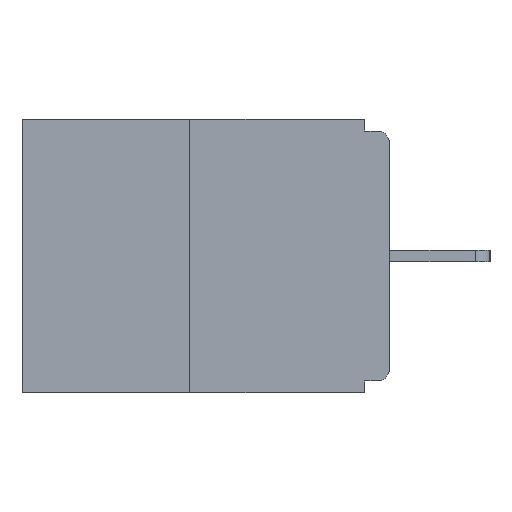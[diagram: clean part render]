
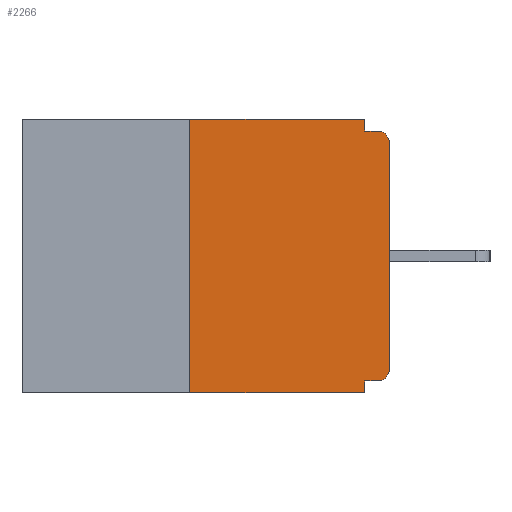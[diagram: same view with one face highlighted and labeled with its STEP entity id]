
A CAD part, left-side view. The second image highlights one B-rep face of the part: STEP entity #2266.
In plain terms, the highlighted planar face has unit normal (-1, 0, 0).
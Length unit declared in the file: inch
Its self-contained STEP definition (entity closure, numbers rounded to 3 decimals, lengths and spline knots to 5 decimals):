
#65 = EDGE_CURVE ( 'NONE', #19768, #17656, #17160, .T. ) ;
#498 = VERTEX_POINT ( 'NONE', #9964 ) ;
#1561 = DIRECTION ( 'NONE',  ( 0., 0., 1. ) ) ;
#2215 = ORIENTED_EDGE ( 'NONE', *, *, #4279, .T. ) ;
#2250 = VERTEX_POINT ( 'NONE', #8593 ) ;
#2266 = ADVANCED_FACE ( 'NONE', ( #8035 ), #17076, .F. ) ;
#3750 = EDGE_CURVE ( 'NONE', #2250, #498, #4359, .T. ) ;
#3853 = CARTESIAN_POINT ( 'NONE',  ( 0., 0.031, -0.328 ) ) ;
#3857 = DIRECTION ( 'NONE',  ( 1., 0., 0. ) ) ;
#4024 = AXIS2_PLACEMENT_3D ( 'NONE', #25520, #3857, #18879 ) ;
#4279 = EDGE_CURVE ( 'NONE', #18692, #2250, #9939, .T. ) ;
#4333 = EDGE_CURVE ( 'NONE', #14753, #22652, #13952, .T. ) ;
#4359 = CIRCLE ( 'NONE', #23442, 0.015 ) ;
#4551 = CARTESIAN_POINT ( 'NONE',  ( 0., 0., -0.015 ) ) ;
#4569 = EDGE_CURVE ( 'NONE', #14753, #17118, #5358, .T. ) ;
#4645 = EDGE_CURVE ( 'NONE', #17656, #498, #15135, .T. ) ;
#4673 = DIRECTION ( 'NONE',  ( -1., 0., 0. ) ) ;
#5358 = LINE ( 'NONE', #18330, #16076 ) ;
#5382 = VECTOR ( 'NONE', #1561, 39.37008 ) ;
#5445 = CARTESIAN_POINT ( 'NONE',  ( 0., 0.015, -0.313 ) ) ;
#6482 = CARTESIAN_POINT ( 'NONE',  ( 0., 0.46, 0. ) ) ;
#6751 = CARTESIAN_POINT ( 'NONE',  ( 0., 0.031, -0.343 ) ) ;
#7049 = CARTESIAN_POINT ( 'NONE',  ( 0., 0.25, -0.343 ) ) ;
#7251 = CARTESIAN_POINT ( 'NONE',  ( 0., 0.015, -0.328 ) ) ;
#7298 = DIRECTION ( 'NONE',  ( 0., 0., 1. ) ) ;
#7662 = ORIENTED_EDGE ( 'NONE', *, *, #65, .F. ) ;
#8035 = FACE_OUTER_BOUND ( 'NONE', #9045, .T. ) ;
#8593 = CARTESIAN_POINT ( 'NONE',  ( 0., 0., -0.03 ) ) ;
#8756 = ORIENTED_EDGE ( 'NONE', *, *, #3750, .T. ) ;
#9045 = EDGE_LOOP ( 'NONE', ( #25460, #13116, #10959, #24243, #26529, #23809, #2215, #8756, #13573, #7662 ) ) ;
#9939 = LINE ( 'NONE', #20631, #5382 ) ;
#9964 = CARTESIAN_POINT ( 'NONE',  ( 0., 0.015, -0.015 ) ) ;
#10185 = CARTESIAN_POINT ( 'NONE',  ( 0., 0.031, 0. ) ) ;
#10533 = LINE ( 'NONE', #6482, #20190 ) ;
#10557 = CIRCLE ( 'NONE', #19886, 0.015 ) ;
#10936 = DIRECTION ( 'NONE',  ( 0., 0., -1. ) ) ;
#10959 = ORIENTED_EDGE ( 'NONE', *, *, #4333, .T. ) ;
#12269 = DIRECTION ( 'NONE',  ( 0., -1., 0. ) ) ;
#12533 = CARTESIAN_POINT ( 'NONE',  ( 0., 0.25, 0. ) ) ;
#12976 = DIRECTION ( 'NONE',  ( 0., 1., 0. ) ) ;
#13116 = ORIENTED_EDGE ( 'NONE', *, *, #4569, .F. ) ;
#13355 = VECTOR ( 'NONE', #21061, 39.37008 ) ;
#13573 = ORIENTED_EDGE ( 'NONE', *, *, #4645, .F. ) ;
#13926 = DIRECTION ( 'NONE',  ( 0., 0., -1. ) ) ;
#13952 = LINE ( 'NONE', #14377, #16057 ) ;
#14137 = EDGE_CURVE ( 'NONE', #14939, #22652, #14802, .T. ) ;
#14377 = CARTESIAN_POINT ( 'NONE',  ( 0., 0.46, -0.343 ) ) ;
#14753 = VERTEX_POINT ( 'NONE', #7049 ) ;
#14802 = LINE ( 'NONE', #6751, #20365 ) ;
#14939 = VERTEX_POINT ( 'NONE', #3853 ) ;
#15135 = LINE ( 'NONE', #4551, #20511 ) ;
#15551 = DIRECTION ( 'NONE',  ( 0., 0., -1. ) ) ;
#16057 = VECTOR ( 'NONE', #12269, 39.37008 ) ;
#16076 = VECTOR ( 'NONE', #7298, 39.37008 ) ;
#17076 = PLANE ( 'NONE',  #4024 ) ;
#17118 = VERTEX_POINT ( 'NONE', #12533 ) ;
#17160 = LINE ( 'NONE', #23120, #13355 ) ;
#17519 = EDGE_CURVE ( 'NONE', #17118, #19768, #10533, .T. ) ;
#17656 = VERTEX_POINT ( 'NONE', #17910 ) ;
#17910 = CARTESIAN_POINT ( 'NONE',  ( 0., 0.031, -0.015 ) ) ;
#18330 = CARTESIAN_POINT ( 'NONE',  ( 0., 0.25, 0. ) ) ;
#18692 = VERTEX_POINT ( 'NONE', #24670 ) ;
#18879 = DIRECTION ( 'NONE',  ( 0., 0., -1. ) ) ;
#19296 = DIRECTION ( 'NONE',  ( 0., -1., 0. ) ) ;
#19768 = VERTEX_POINT ( 'NONE', #10185 ) ;
#19886 = AXIS2_PLACEMENT_3D ( 'NONE', #5445, #24620, #13926 ) ;
#20190 = VECTOR ( 'NONE', #23572, 39.37008 ) ;
#20365 = VECTOR ( 'NONE', #10936, 39.37008 ) ;
#20511 = VECTOR ( 'NONE', #19296, 39.37008 ) ;
#20631 = CARTESIAN_POINT ( 'NONE',  ( 0., 0., 0. ) ) ;
#21061 = DIRECTION ( 'NONE',  ( 0., 0., -1. ) ) ;
#21798 = CARTESIAN_POINT ( 'NONE',  ( 0., 0.015, -0.03 ) ) ;
#21947 = VERTEX_POINT ( 'NONE', #7251 ) ;
#22040 = EDGE_CURVE ( 'NONE', #21947, #18692, #10557, .T. ) ;
#22586 = VECTOR ( 'NONE', #12976, 39.37008 ) ;
#22652 = VERTEX_POINT ( 'NONE', #23604 ) ;
#23120 = CARTESIAN_POINT ( 'NONE',  ( 0., 0.031, 0. ) ) ;
#23442 = AXIS2_PLACEMENT_3D ( 'NONE', #21798, #4673, #15551 ) ;
#23572 = DIRECTION ( 'NONE',  ( 0., -1., 0. ) ) ;
#23604 = CARTESIAN_POINT ( 'NONE',  ( 0., 0.031, -0.343 ) ) ;
#23809 = ORIENTED_EDGE ( 'NONE', *, *, #22040, .T. ) ;
#23968 = LINE ( 'NONE', #26039, #22586 ) ;
#24243 = ORIENTED_EDGE ( 'NONE', *, *, #14137, .F. ) ;
#24620 = DIRECTION ( 'NONE',  ( -1., 0., 0. ) ) ;
#24670 = CARTESIAN_POINT ( 'NONE',  ( 0., 0., -0.313 ) ) ;
#25460 = ORIENTED_EDGE ( 'NONE', *, *, #17519, .F. ) ;
#25520 = CARTESIAN_POINT ( 'NONE',  ( 0., 0.46, 0. ) ) ;
#26039 = CARTESIAN_POINT ( 'NONE',  ( 0., 0., -0.328 ) ) ;
#26529 = ORIENTED_EDGE ( 'NONE', *, *, #27351, .F. ) ;
#27351 = EDGE_CURVE ( 'NONE', #21947, #14939, #23968, .T. ) ;
